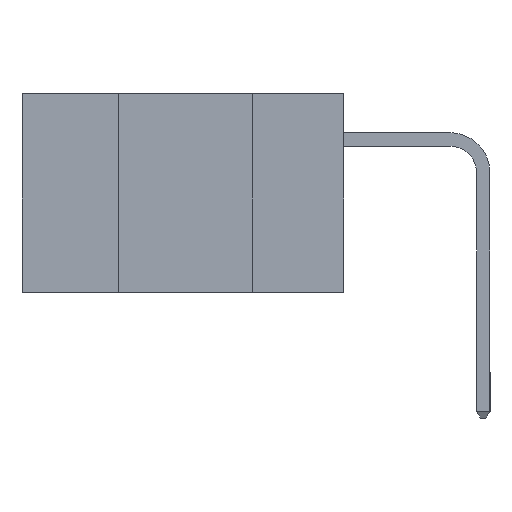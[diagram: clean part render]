
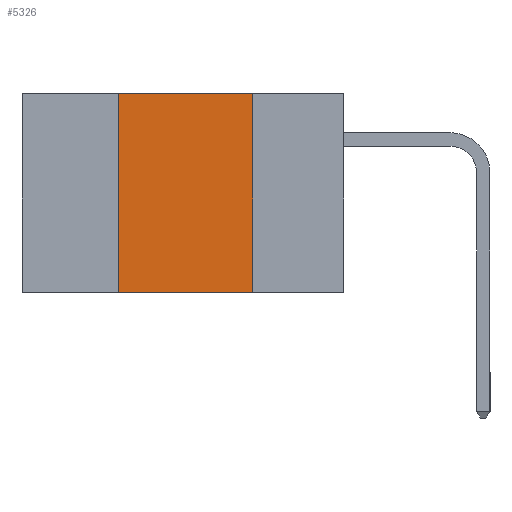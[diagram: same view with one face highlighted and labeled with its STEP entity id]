
A CAD part, left-side view. The second image highlights one B-rep face of the part: STEP entity #5326.
In plain terms, the highlighted planar face has unit normal (-1, 0, 0).
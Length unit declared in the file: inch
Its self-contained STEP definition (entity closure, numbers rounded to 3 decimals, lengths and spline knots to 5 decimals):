
#96 = LINE ( 'NONE', #3321, #1613 ) ;
#386 = CARTESIAN_POINT ( 'NONE',  ( 0., 0.6, 0. ) ) ;
#442 = PLANE ( 'NONE',  #4166 ) ;
#1464 = CARTESIAN_POINT ( 'NONE',  ( 0., 0.17, 0. ) ) ;
#1573 = EDGE_CURVE ( 'NONE', #11898, #4260, #2817, .T. ) ;
#1613 = VECTOR ( 'NONE', #9996, 39.37008 ) ;
#2231 = ORIENTED_EDGE ( 'NONE', *, *, #6792, .F. ) ;
#2292 = EDGE_CURVE ( 'NONE', #11898, #6838, #96, .T. ) ;
#2358 = EDGE_CURVE ( 'NONE', #8638, #6838, #8004, .T. ) ;
#2817 = LINE ( 'NONE', #4931, #12055 ) ;
#3321 = CARTESIAN_POINT ( 'NONE',  ( 0., 0.6, -0.37 ) ) ;
#3404 = DIRECTION ( 'NONE',  ( 0., 0., -1. ) ) ;
#3756 = EDGE_LOOP ( 'NONE', ( #4413, #2231, #6581, #8668 ) ) ;
#4096 = VECTOR ( 'NONE', #8068, 39.37008 ) ;
#4166 = AXIS2_PLACEMENT_3D ( 'NONE', #9077, #6254, #7131 ) ;
#4260 = VERTEX_POINT ( 'NONE', #8268 ) ;
#4413 = ORIENTED_EDGE ( 'NONE', *, *, #2358, .F. ) ;
#4931 = CARTESIAN_POINT ( 'NONE',  ( 0., 0.42, 0. ) ) ;
#5326 = ADVANCED_FACE ( 'NONE', ( #6278 ), #442, .F. ) ;
#6254 = DIRECTION ( 'NONE',  ( 1., 0., 0. ) ) ;
#6278 = FACE_OUTER_BOUND ( 'NONE', #3756, .T. ) ;
#6581 = ORIENTED_EDGE ( 'NONE', *, *, #1573, .F. ) ;
#6792 = EDGE_CURVE ( 'NONE', #4260, #8638, #7519, .T. ) ;
#6838 = VERTEX_POINT ( 'NONE', #7072 ) ;
#6842 = DIRECTION ( 'NONE',  ( 0., 0., 1. ) ) ;
#7072 = CARTESIAN_POINT ( 'NONE',  ( 0., 0.17, -0.37 ) ) ;
#7131 = DIRECTION ( 'NONE',  ( 0., 0., -1. ) ) ;
#7282 = VECTOR ( 'NONE', #3404, 39.37008 ) ;
#7519 = LINE ( 'NONE', #386, #4096 ) ;
#8004 = LINE ( 'NONE', #1464, #7282 ) ;
#8068 = DIRECTION ( 'NONE',  ( 0., -1., 0. ) ) ;
#8268 = CARTESIAN_POINT ( 'NONE',  ( 0., 0.42, 0. ) ) ;
#8638 = VERTEX_POINT ( 'NONE', #11799 ) ;
#8668 = ORIENTED_EDGE ( 'NONE', *, *, #2292, .T. ) ;
#9077 = CARTESIAN_POINT ( 'NONE',  ( 0., 0.6, 0. ) ) ;
#9996 = DIRECTION ( 'NONE',  ( 0., -1., 0. ) ) ;
#11381 = CARTESIAN_POINT ( 'NONE',  ( 0., 0.42, -0.37 ) ) ;
#11799 = CARTESIAN_POINT ( 'NONE',  ( 0., 0.17, 0. ) ) ;
#11898 = VERTEX_POINT ( 'NONE', #11381 ) ;
#12055 = VECTOR ( 'NONE', #6842, 39.37008 ) ;
